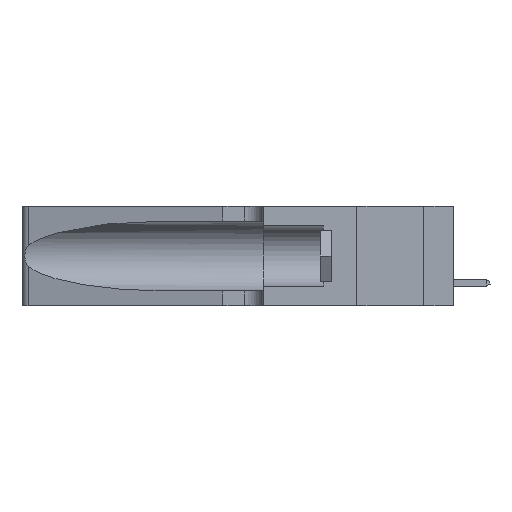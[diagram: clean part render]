
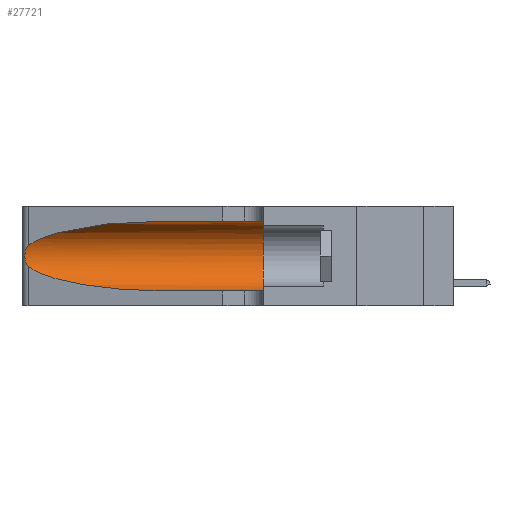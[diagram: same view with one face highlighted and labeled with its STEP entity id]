
A CAD part, left-side view. The second image highlights one B-rep face of the part: STEP entity #27721.
In plain terms, the highlighted cylindrical face has radius 3.308 mm (diameter 6.617 mm), a partial arc.
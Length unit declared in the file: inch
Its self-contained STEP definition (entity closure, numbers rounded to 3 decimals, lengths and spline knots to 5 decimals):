
#1446 = EDGE_CURVE ( 'NONE', #25538, #24941, #22202, .T. ) ;
#2213 = CARTESIAN_POINT ( 'NONE',  ( 0.25787, 1.23484, 0.2124 ) ) ;
#2734 = CARTESIAN_POINT ( 'NONE',  ( 0.25487, 1.22718, 0.14631 ) ) ;
#4303 = CARTESIAN_POINT ( 'NONE',  ( 0.25555, 1.22993, 0.14849 ) ) ;
#4349 = EDGE_CURVE ( 'NONE', #30789, #25538, #14762, .T. ) ;
#4458 = CARTESIAN_POINT ( 'NONE',  ( 0.18966, 0.96281, 0.05475 ) ) ;
#5447 = EDGE_CURVE ( 'NONE', #9493, #13598, #12260, .T. ) ;
#5506 = DIRECTION ( 'NONE',  ( 0., 0., -1. ) ) ;
#6352 = ORIENTED_EDGE ( 'NONE', *, *, #1446, .T. ) ;
#6703 = CARTESIAN_POINT ( 'NONE',  ( 0.25487, 1.22718, 0.14631 ) ) ;
#6761 = CARTESIAN_POINT ( 'NONE',  ( 0.25639, 1.23184, 0.21858 ) ) ;
#7337 = ORIENTED_EDGE ( 'NONE', *, *, #5447, .F. ) ;
#7665 = DIRECTION ( 'NONE',  ( 0., -1., 0. ) ) ;
#7986 = CARTESIAN_POINT ( 'NONE',  ( 0.1305, 0.72297, 0.31525 ) ) ;
#8697 = VERTEX_POINT ( 'NONE', #29631 ) ;
#8875 = DIRECTION ( 'NONE',  ( 0., -1., 0. ) ) ;
#8921 = EDGE_CURVE ( 'NONE', #8697, #9493, #28022, .T. ) ;
#8965 = CARTESIAN_POINT ( 'NONE',  ( 0.25789, 1.23486, 0.15765 ) ) ;
#9032 = VECTOR ( 'NONE', #8875, 39.37008 ) ;
#9387 = CARTESIAN_POINT ( 'NONE',  ( 0.25856, 1.23593, 0.16098 ) ) ;
#9493 = VERTEX_POINT ( 'NONE', #14192 ) ;
#9833 = CARTESIAN_POINT ( 'NONE',  ( 0.1305, 0.72297, 0.05475 ) ) ;
#9858 = CARTESIAN_POINT ( 'NONE',  ( 0.1305, 1.61858, 0.05475 ) ) ;
#9887 = CARTESIAN_POINT ( 'NONE',  ( 0.1305, 1.61858, 0.185 ) ) ;
#10359 = ORIENTED_EDGE ( 'NONE', *, *, #8921, .F. ) ;
#10414 = EDGE_CURVE ( 'NONE', #8697, #30789, #18977, .T. ) ;
#11169 = CYLINDRICAL_SURFACE ( 'NONE', #27398, 0.13025 ) ;
#11922 = FACE_OUTER_BOUND ( 'NONE', #16492, .T. ) ;
#11943 = DIRECTION ( 'NONE',  ( 0., -1., 0. ) ) ;
#12260 = CIRCLE ( 'NONE', #20911, 0.13025 ) ;
#12763 = ORIENTED_EDGE ( 'NONE', *, *, #20705, .T. ) ;
#13598 = VERTEX_POINT ( 'NONE', #22668 ) ;
#13988 = CARTESIAN_POINT ( 'NONE',  ( 0.25854, 1.2359, 0.20912 ) ) ;
#14033 = CARTESIAN_POINT ( 'NONE',  ( 0.1305, 0.72297, 0.05475 ) ) ;
#14192 = CARTESIAN_POINT ( 'NONE',  ( 0.1305, 0.35, 0.31525 ) ) ;
#14389 = VECTOR ( 'NONE', #11943, 39.37008 ) ;
#14762 = B_SPLINE_CURVE_WITH_KNOTS ( 'NONE', 3,
 ( #23273, #16503, #6761, #2213, #13988, #18908, #30394, #21272, #30589, #9387, #8965, #18612, #4303, #2734 ),
 .UNSPECIFIED., .F., .F.,
 ( 4, 2, 2, 2, 2, 2, 4 ),
 ( 0., 0.00027, 0.00053, 0.00107, 0.0016, 0.00187, 0.00214 ),
 .UNSPECIFIED. ) ;
#16492 = EDGE_LOOP ( 'NONE', ( #26343, #23998, #6352, #12763, #7337, #10359 ) ) ;
#16503 = CARTESIAN_POINT ( 'NONE',  ( 0.25555, 1.22994, 0.2215 ) ) ;
#17621 = DIRECTION ( 'NONE',  ( 0., 1., 0. ) ) ;
#18612 = CARTESIAN_POINT ( 'NONE',  ( 0.25639, 1.23186, 0.15144 ) ) ;
#18908 = CARTESIAN_POINT ( 'NONE',  ( 0.26018, 1.23835, 0.19895 ) ) ;
#18977 =( BOUNDED_CURVE ( )  B_SPLINE_CURVE ( 3, ( #7986, #20120, #22206, #29339 ),
 .UNSPECIFIED., .F., .F. ) 
 B_SPLINE_CURVE_WITH_KNOTS ( ( 4, 4 ),
 ( 1.5708, 2.84003 ),
 .UNSPECIFIED. ) 
 CURVE ( )  GEOMETRIC_REPRESENTATION_ITEM ( )  RATIONAL_B_SPLINE_CURVE ( ( 1., 0.87, 0.87, 1. ) ) 
 REPRESENTATION_ITEM ( '' )  );
#19178 = CARTESIAN_POINT ( 'NONE',  ( 0.2373, 1.15595, 0.08982 ) ) ;
#20120 = CARTESIAN_POINT ( 'NONE',  ( 0.18966, 0.96281, 0.31525 ) ) ;
#20705 = EDGE_CURVE ( 'NONE', #24941, #13598, #24060, .T. ) ;
#20911 = AXIS2_PLACEMENT_3D ( 'NONE', #27147, #17621, #29526 ) ;
#21272 = CARTESIAN_POINT ( 'NONE',  ( 0.26075, 1.23896, 0.178 ) ) ;
#22202 =( BOUNDED_CURVE ( )  B_SPLINE_CURVE ( 3, ( #6703, #19178, #4458, #14033 ),
 .UNSPECIFIED., .F., .T. ) 
 B_SPLINE_CURVE_WITH_KNOTS ( ( 4, 4 ),
 ( 3.44316, 4.71239 ),
 .UNSPECIFIED. ) 
 CURVE ( )  GEOMETRIC_REPRESENTATION_ITEM ( )  RATIONAL_B_SPLINE_CURVE ( ( 1., 0.87, 0.87, 1. ) ) 
 REPRESENTATION_ITEM ( '' )  );
#22206 = CARTESIAN_POINT ( 'NONE',  ( 0.2373, 1.15595, 0.28018 ) ) ;
#22668 = CARTESIAN_POINT ( 'NONE',  ( 0.1305, 0.35, 0.05475 ) ) ;
#23187 = CARTESIAN_POINT ( 'NONE',  ( 0.1305, 1.61858, 0.31525 ) ) ;
#23273 = CARTESIAN_POINT ( 'NONE',  ( 0.25487, 1.22718, 0.22369 ) ) ;
#23998 = ORIENTED_EDGE ( 'NONE', *, *, #4349, .T. ) ;
#24060 = LINE ( 'NONE', #9858, #14389 ) ;
#24941 = VERTEX_POINT ( 'NONE', #9833 ) ;
#25515 = CARTESIAN_POINT ( 'NONE',  ( 0.25487, 1.22718, 0.14631 ) ) ;
#25538 = VERTEX_POINT ( 'NONE', #25515 ) ;
#26343 = ORIENTED_EDGE ( 'NONE', *, *, #10414, .T. ) ;
#27147 = CARTESIAN_POINT ( 'NONE',  ( 0.1305, 0.35, 0.185 ) ) ;
#27398 = AXIS2_PLACEMENT_3D ( 'NONE', #9887, #7665, #5506 ) ;
#27721 = ADVANCED_FACE ( 'NONE', ( #11922 ), #11169, .F. ) ;
#28022 = LINE ( 'NONE', #23187, #9032 ) ;
#29339 = CARTESIAN_POINT ( 'NONE',  ( 0.25487, 1.22718, 0.22369 ) ) ;
#29526 = DIRECTION ( 'NONE',  ( 0., 0., 1. ) ) ;
#29631 = CARTESIAN_POINT ( 'NONE',  ( 0.1305, 0.72297, 0.31525 ) ) ;
#30394 = CARTESIAN_POINT ( 'NONE',  ( 0.26075, 1.23896, 0.19203 ) ) ;
#30589 = CARTESIAN_POINT ( 'NONE',  ( 0.26017, 1.23833, 0.17102 ) ) ;
#30789 = VERTEX_POINT ( 'NONE', #30806 ) ;
#30806 = CARTESIAN_POINT ( 'NONE',  ( 0.25487, 1.22718, 0.22369 ) ) ;
